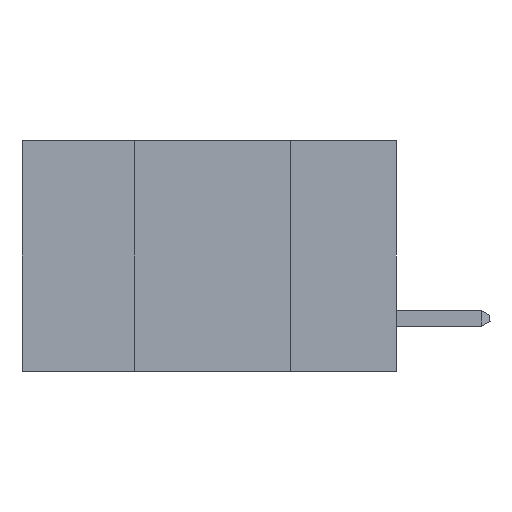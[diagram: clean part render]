
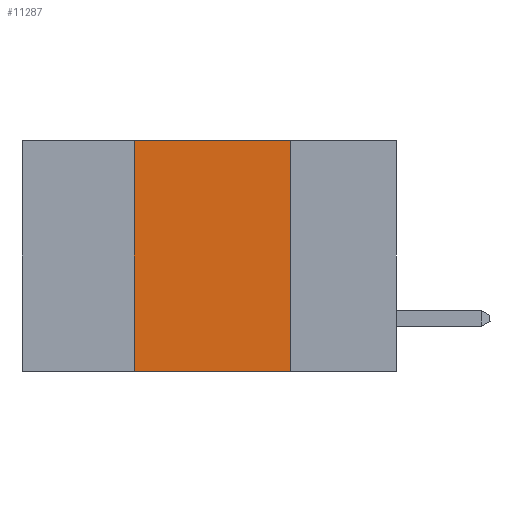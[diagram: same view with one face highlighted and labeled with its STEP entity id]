
A CAD part, left-side view. The second image highlights one B-rep face of the part: STEP entity #11287.
In plain terms, the highlighted planar face has unit normal (-1, 0, 0).
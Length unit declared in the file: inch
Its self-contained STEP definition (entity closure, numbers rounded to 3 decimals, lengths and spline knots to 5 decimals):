
#106 = VECTOR ( 'NONE', #10707, 39.37008 ) ;
#261 = ORIENTED_EDGE ( 'NONE', *, *, #9869, .F. ) ;
#310 = VERTEX_POINT ( 'NONE', #7951 ) ;
#1628 = EDGE_CURVE ( 'NONE', #4078, #6486, #10933, .T. ) ;
#2204 = PLANE ( 'NONE',  #11502 ) ;
#2380 = DIRECTION ( 'NONE',  ( 0., 0., -1. ) ) ;
#2483 = ORIENTED_EDGE ( 'NONE', *, *, #3514, .F. ) ;
#2827 = LINE ( 'NONE', #7805, #106 ) ;
#3138 = VECTOR ( 'NONE', #2380, 39.37008 ) ;
#3514 = EDGE_CURVE ( 'NONE', #5282, #4078, #11732, .T. ) ;
#3869 = CARTESIAN_POINT ( 'NONE',  ( 0., 0.6, -0.37 ) ) ;
#3950 = CARTESIAN_POINT ( 'NONE',  ( 0., 0.17, 0. ) ) ;
#4066 = CARTESIAN_POINT ( 'NONE',  ( 0., 0.42, 0. ) ) ;
#4078 = VERTEX_POINT ( 'NONE', #10439 ) ;
#4084 = CARTESIAN_POINT ( 'NONE',  ( 0., 0.6, 0. ) ) ;
#5130 = CARTESIAN_POINT ( 'NONE',  ( 0., 0.6, 0. ) ) ;
#5282 = VERTEX_POINT ( 'NONE', #4066 ) ;
#5735 = VECTOR ( 'NONE', #11360, 39.37008 ) ;
#6014 = DIRECTION ( 'NONE',  ( 0., 0., -1. ) ) ;
#6486 = VERTEX_POINT ( 'NONE', #10930 ) ;
#7130 = FACE_OUTER_BOUND ( 'NONE', #11097, .T. ) ;
#7148 = ORIENTED_EDGE ( 'NONE', *, *, #1628, .F. ) ;
#7595 = LINE ( 'NONE', #3869, #5735 ) ;
#7805 = CARTESIAN_POINT ( 'NONE',  ( 0., 0.42, 0. ) ) ;
#7951 = CARTESIAN_POINT ( 'NONE',  ( 0., 0.42, -0.37 ) ) ;
#8293 = ORIENTED_EDGE ( 'NONE', *, *, #11079, .T. ) ;
#8745 = DIRECTION ( 'NONE',  ( 0., -1., 0. ) ) ;
#9348 = VECTOR ( 'NONE', #8745, 39.37008 ) ;
#9869 = EDGE_CURVE ( 'NONE', #310, #5282, #2827, .T. ) ;
#10439 = CARTESIAN_POINT ( 'NONE',  ( 0., 0.17, 0. ) ) ;
#10707 = DIRECTION ( 'NONE',  ( 0., 0., 1. ) ) ;
#10930 = CARTESIAN_POINT ( 'NONE',  ( 0., 0.17, -0.37 ) ) ;
#10933 = LINE ( 'NONE', #3950, #3138 ) ;
#11079 = EDGE_CURVE ( 'NONE', #310, #6486, #7595, .T. ) ;
#11097 = EDGE_LOOP ( 'NONE', ( #7148, #2483, #261, #8293 ) ) ;
#11287 = ADVANCED_FACE ( 'NONE', ( #7130 ), #2204, .F. ) ;
#11360 = DIRECTION ( 'NONE',  ( 0., -1., 0. ) ) ;
#11502 = AXIS2_PLACEMENT_3D ( 'NONE', #5130, #11660, #6014 ) ;
#11660 = DIRECTION ( 'NONE',  ( 1., 0., 0. ) ) ;
#11732 = LINE ( 'NONE', #4084, #9348 ) ;
